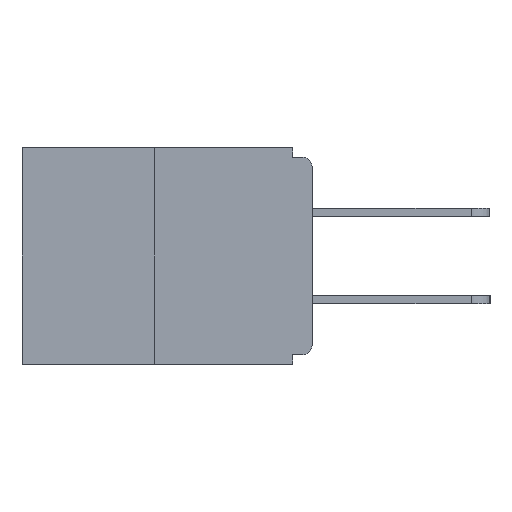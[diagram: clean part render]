
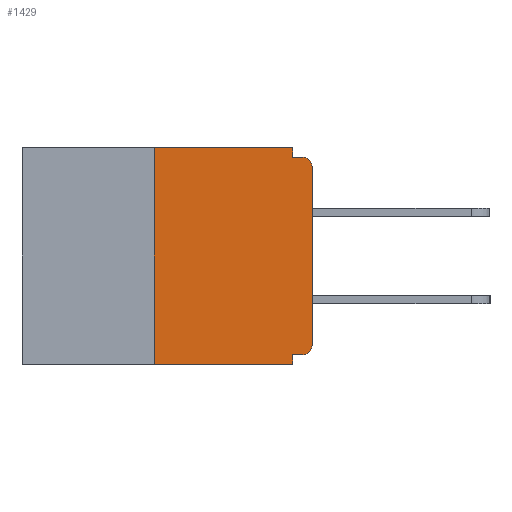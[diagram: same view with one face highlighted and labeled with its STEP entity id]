
A CAD part, left-side view. The second image highlights one B-rep face of the part: STEP entity #1429.
In plain terms, the highlighted planar face has unit normal (-1, 0, 0).
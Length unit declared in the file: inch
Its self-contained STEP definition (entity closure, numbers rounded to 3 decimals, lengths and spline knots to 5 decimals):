
#26 = DIRECTION ( 'NONE',  ( 1., 0., 0. ) ) ;
#241 = EDGE_CURVE ( 'NONE', #2928, #3564, #12528, .T. ) ;
#261 = CARTESIAN_POINT ( 'NONE',  ( 0., 0.015, -0.015 ) ) ;
#484 = VECTOR ( 'NONE', #3970, 39.37008 ) ;
#853 = LINE ( 'NONE', #7533, #2188 ) ;
#886 = DIRECTION ( 'NONE',  ( 0., 0., -1. ) ) ;
#1429 = ADVANCED_FACE ( 'NONE', ( #10378 ), #14771, .F. ) ;
#2188 = VECTOR ( 'NONE', #2840, 39.37008 ) ;
#2285 = DIRECTION ( 'NONE',  ( 0., 0., -1. ) ) ;
#2439 = CARTESIAN_POINT ( 'NONE',  ( 0., 0.46, 0. ) ) ;
#2458 = ORIENTED_EDGE ( 'NONE', *, *, #12211, .F. ) ;
#2633 = EDGE_LOOP ( 'NONE', ( #5850, #12678, #9640, #12781, #8687, #7835, #3016, #9532, #15416, #2458 ) ) ;
#2840 = DIRECTION ( 'NONE',  ( 0., 0., -1. ) ) ;
#2928 = VERTEX_POINT ( 'NONE', #6515 ) ;
#3016 = ORIENTED_EDGE ( 'NONE', *, *, #10717, .T. ) ;
#3197 = VECTOR ( 'NONE', #5111, 39.37008 ) ;
#3312 = DIRECTION ( 'NONE',  ( -1., 0., 0. ) ) ;
#3380 = EDGE_CURVE ( 'NONE', #11198, #9377, #13335, .T. ) ;
#3447 = VERTEX_POINT ( 'NONE', #11492 ) ;
#3564 = VERTEX_POINT ( 'NONE', #5341 ) ;
#3888 = VECTOR ( 'NONE', #8679, 39.37008 ) ;
#3970 = DIRECTION ( 'NONE',  ( 0., -1., 0. ) ) ;
#3976 = VERTEX_POINT ( 'NONE', #6741 ) ;
#5111 = DIRECTION ( 'NONE',  ( 0., 0., -1. ) ) ;
#5195 = CARTESIAN_POINT ( 'NONE',  ( 0., 0., -0.328 ) ) ;
#5280 = VERTEX_POINT ( 'NONE', #8102 ) ;
#5341 = CARTESIAN_POINT ( 'NONE',  ( 0., 0.031, 0. ) ) ;
#5576 = CARTESIAN_POINT ( 'NONE',  ( 0., 0.25, 0. ) ) ;
#5741 = VERTEX_POINT ( 'NONE', #261 ) ;
#5850 = ORIENTED_EDGE ( 'NONE', *, *, #241, .F. ) ;
#6078 = DIRECTION ( 'NONE',  ( 0., 0., -1. ) ) ;
#6089 = CARTESIAN_POINT ( 'NONE',  ( 0., 0.46, 0. ) ) ;
#6515 = CARTESIAN_POINT ( 'NONE',  ( 0., 0.25, 0. ) ) ;
#6591 = AXIS2_PLACEMENT_3D ( 'NONE', #14424, #3312, #886 ) ;
#6741 = CARTESIAN_POINT ( 'NONE',  ( 0., 0.031, -0.015 ) ) ;
#6961 = CARTESIAN_POINT ( 'NONE',  ( 0., 0.015, -0.328 ) ) ;
#7014 = CIRCLE ( 'NONE', #6591, 0.015 ) ;
#7083 = LINE ( 'NONE', #5576, #13999 ) ;
#7215 = LINE ( 'NONE', #5195, #14497 ) ;
#7336 = EDGE_CURVE ( 'NONE', #8716, #12209, #7215, .T. ) ;
#7533 = CARTESIAN_POINT ( 'NONE',  ( 0., 0.031, 0. ) ) ;
#7671 = EDGE_CURVE ( 'NONE', #5280, #5741, #7014, .T. ) ;
#7819 = LINE ( 'NONE', #13894, #484 ) ;
#7835 = ORIENTED_EDGE ( 'NONE', *, *, #13983, .T. ) ;
#8102 = CARTESIAN_POINT ( 'NONE',  ( 0., 0., -0.03 ) ) ;
#8679 = DIRECTION ( 'NONE',  ( 0., -1., 0. ) ) ;
#8687 = ORIENTED_EDGE ( 'NONE', *, *, #7336, .F. ) ;
#8695 = CARTESIAN_POINT ( 'NONE',  ( 0., 0.031, -0.328 ) ) ;
#8716 = VERTEX_POINT ( 'NONE', #6961 ) ;
#8875 = CARTESIAN_POINT ( 'NONE',  ( 0., 0., 0. ) ) ;
#9023 = DIRECTION ( 'NONE',  ( 0., 0., 1. ) ) ;
#9377 = VERTEX_POINT ( 'NONE', #10694 ) ;
#9532 = ORIENTED_EDGE ( 'NONE', *, *, #7671, .T. ) ;
#9640 = ORIENTED_EDGE ( 'NONE', *, *, #3380, .T. ) ;
#9740 = DIRECTION ( 'NONE',  ( -1., 0., 0. ) ) ;
#9941 = LINE ( 'NONE', #8875, #10712 ) ;
#9946 = EDGE_CURVE ( 'NONE', #11198, #2928, #7083, .T. ) ;
#10378 = FACE_OUTER_BOUND ( 'NONE', #2633, .T. ) ;
#10625 = EDGE_CURVE ( 'NONE', #12209, #9377, #13589, .T. ) ;
#10653 = EDGE_CURVE ( 'NONE', #3976, #5741, #7819, .T. ) ;
#10694 = CARTESIAN_POINT ( 'NONE',  ( 0., 0.031, -0.343 ) ) ;
#10712 = VECTOR ( 'NONE', #9023, 39.37008 ) ;
#10717 = EDGE_CURVE ( 'NONE', #3447, #5280, #9941, .T. ) ;
#10910 = AXIS2_PLACEMENT_3D ( 'NONE', #2439, #26, #2285 ) ;
#10943 = DIRECTION ( 'NONE',  ( 0., -1., 0. ) ) ;
#11198 = VERTEX_POINT ( 'NONE', #14261 ) ;
#11492 = CARTESIAN_POINT ( 'NONE',  ( 0., 0., -0.313 ) ) ;
#12209 = VERTEX_POINT ( 'NONE', #8695 ) ;
#12211 = EDGE_CURVE ( 'NONE', #3564, #3976, #853, .T. ) ;
#12528 = LINE ( 'NONE', #6089, #13291 ) ;
#12626 = DIRECTION ( 'NONE',  ( 0., 1., 0. ) ) ;
#12678 = ORIENTED_EDGE ( 'NONE', *, *, #9946, .F. ) ;
#12781 = ORIENTED_EDGE ( 'NONE', *, *, #10625, .F. ) ;
#12986 = AXIS2_PLACEMENT_3D ( 'NONE', #13344, #9740, #6078 ) ;
#13291 = VECTOR ( 'NONE', #10943, 39.37008 ) ;
#13335 = LINE ( 'NONE', #15020, #3888 ) ;
#13344 = CARTESIAN_POINT ( 'NONE',  ( 0., 0.015, -0.313 ) ) ;
#13589 = LINE ( 'NONE', #15104, #3197 ) ;
#13894 = CARTESIAN_POINT ( 'NONE',  ( 0., 0., -0.015 ) ) ;
#13983 = EDGE_CURVE ( 'NONE', #8716, #3447, #15848, .T. ) ;
#13999 = VECTOR ( 'NONE', #14269, 39.37008 ) ;
#14261 = CARTESIAN_POINT ( 'NONE',  ( 0., 0.25, -0.343 ) ) ;
#14269 = DIRECTION ( 'NONE',  ( 0., 0., 1. ) ) ;
#14424 = CARTESIAN_POINT ( 'NONE',  ( 0., 0.015, -0.03 ) ) ;
#14497 = VECTOR ( 'NONE', #12626, 39.37008 ) ;
#14771 = PLANE ( 'NONE',  #10910 ) ;
#15020 = CARTESIAN_POINT ( 'NONE',  ( 0., 0.46, -0.343 ) ) ;
#15104 = CARTESIAN_POINT ( 'NONE',  ( 0., 0.031, -0.343 ) ) ;
#15416 = ORIENTED_EDGE ( 'NONE', *, *, #10653, .F. ) ;
#15848 = CIRCLE ( 'NONE', #12986, 0.015 ) ;
